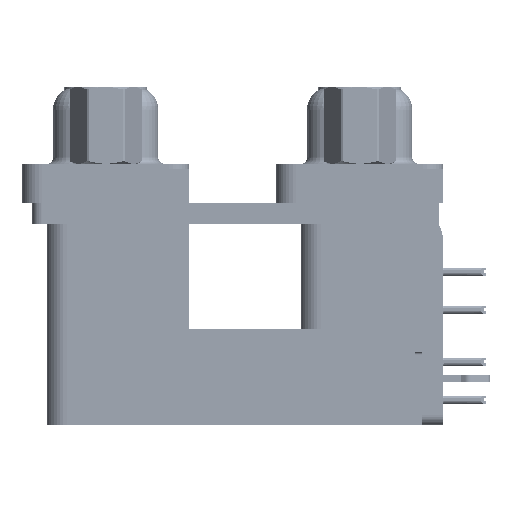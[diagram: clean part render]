
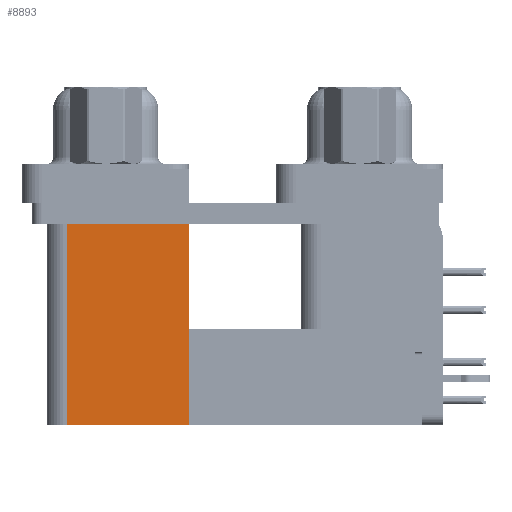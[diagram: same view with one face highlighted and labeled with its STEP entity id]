
A CAD part, left-side view. The second image highlights one B-rep face of the part: STEP entity #8893.
In plain terms, the highlighted planar face has unit normal (-1, 0, 0).
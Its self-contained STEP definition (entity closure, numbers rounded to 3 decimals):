
#3300 = CARTESIAN_POINT ( 'NONE',  ( 3.79, 12.775, -19.2 ) ) ;
#5956 = DIRECTION ( 'NONE',  ( 0., 1., 0. ) ) ;
#6590 = EDGE_CURVE ( 'NONE', #76319, #49883, #49490, .T. ) ;
#8893 = ADVANCED_FACE ( 'NONE', ( #19078 ), #57203, .F. ) ;
#10154 = DIRECTION ( 'NONE',  ( 0., 0., 1. ) ) ;
#11370 = LINE ( 'NONE', #61842, #30385 ) ;
#15260 = LINE ( 'NONE', #3300, #47982 ) ;
#19078 = FACE_OUTER_BOUND ( 'NONE', #75808, .T. ) ;
#27949 = CARTESIAN_POINT ( 'NONE',  ( 3.79, 12.775, -19.2 ) ) ;
#28071 = EDGE_CURVE ( 'NONE', #50585, #49883, #11370, .T. ) ;
#28085 = LINE ( 'NONE', #28485, #33518 ) ;
#28378 = DIRECTION ( 'NONE',  ( 0., 1., 0. ) ) ;
#28485 = CARTESIAN_POINT ( 'NONE',  ( 3.79, 12.775, -19.2 ) ) ;
#29570 = ORIENTED_EDGE ( 'NONE', *, *, #6590, .T. ) ;
#30385 = VECTOR ( 'NONE', #10154, 1000. ) ;
#33518 = VECTOR ( 'NONE', #53122, 1000. ) ;
#35087 = EDGE_CURVE ( 'NONE', #68253, #76319, #28085, .T. ) ;
#36139 = ORIENTED_EDGE ( 'NONE', *, *, #55161, .F. ) ;
#37179 = CARTESIAN_POINT ( 'NONE',  ( 3.79, 12.775, -2.5 ) ) ;
#43420 = VECTOR ( 'NONE', #5956, 1000. ) ;
#44480 = ORIENTED_EDGE ( 'NONE', *, *, #35087, .T. ) ;
#47982 = VECTOR ( 'NONE', #28378, 1000. ) ;
#49490 = LINE ( 'NONE', #37179, #43420 ) ;
#49883 = VERTEX_POINT ( 'NONE', #73159 ) ;
#50585 = VERTEX_POINT ( 'NONE', #58606 ) ;
#51051 = DIRECTION ( 'NONE',  ( 1., 0., 0. ) ) ;
#53122 = DIRECTION ( 'NONE',  ( 0., 0., 1. ) ) ;
#55161 = EDGE_CURVE ( 'NONE', #68253, #50585, #15260, .T. ) ;
#55354 = CARTESIAN_POINT ( 'NONE',  ( 3.79, 12.775, -2.5 ) ) ;
#55911 = ORIENTED_EDGE ( 'NONE', *, *, #28071, .F. ) ;
#56796 = CARTESIAN_POINT ( 'NONE',  ( 3.79, 12.775, -19.2 ) ) ;
#57203 = PLANE ( 'NONE',  #57285 ) ;
#57285 = AXIS2_PLACEMENT_3D ( 'NONE', #56796, #51051, #69136 ) ;
#58606 = CARTESIAN_POINT ( 'NONE',  ( 3.79, 21.975, -19.2 ) ) ;
#61842 = CARTESIAN_POINT ( 'NONE',  ( 3.79, 21.975, -19.2 ) ) ;
#68253 = VERTEX_POINT ( 'NONE', #27949 ) ;
#69136 = DIRECTION ( 'NONE',  ( 0., 0., -1. ) ) ;
#73159 = CARTESIAN_POINT ( 'NONE',  ( 3.79, 21.975, -2.5 ) ) ;
#75808 = EDGE_LOOP ( 'NONE', ( #29570, #55911, #36139, #44480 ) ) ;
#76319 = VERTEX_POINT ( 'NONE', #55354 ) ;
